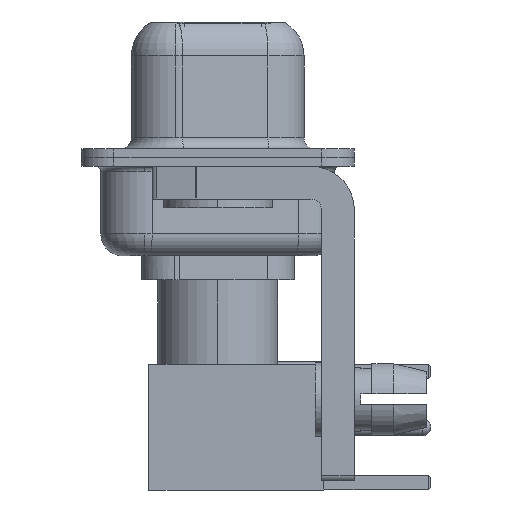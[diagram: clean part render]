
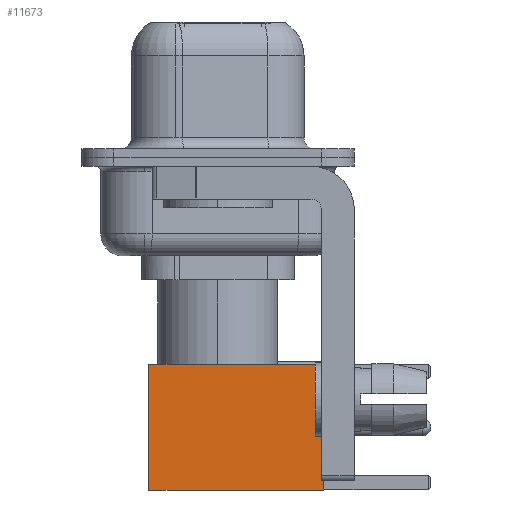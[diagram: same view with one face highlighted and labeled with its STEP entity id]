
A CAD part, left-side view. The second image highlights one B-rep face of the part: STEP entity #11673.
In plain terms, the highlighted face is planar.
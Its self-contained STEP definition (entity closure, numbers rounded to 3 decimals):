
#949 = EDGE_CURVE ( 'NONE', #5847, #16238, #15309, .T. ) ;
#1483 = VERTEX_POINT ( 'NONE', #9457 ) ;
#2577 = CARTESIAN_POINT ( 'NONE',  ( 2.875, 2.875, 0. ) ) ;
#3178 = AXIS2_PLACEMENT_3D ( 'NONE', #21093, #12056, #19308 ) ;
#4596 = EDGE_CURVE ( 'NONE', #1483, #5847, #5017, .T. ) ;
#5017 = LINE ( 'NONE', #12324, #17441 ) ;
#5847 = VERTEX_POINT ( 'NONE', #8816 ) ;
#6822 = ORIENTED_EDGE ( 'NONE', *, *, #949, .F. ) ;
#7757 = LINE ( 'NONE', #15028, #9255 ) ;
#8816 = CARTESIAN_POINT ( 'NONE',  ( -2.875, 2.875, 8. ) ) ;
#9255 = VECTOR ( 'NONE', #9787, 1000. ) ;
#9457 = CARTESIAN_POINT ( 'NONE',  ( 2.875, 2.875, 8. ) ) ;
#9787 = DIRECTION ( 'NONE',  ( -1., 0., 0. ) ) ;
#10222 = EDGE_CURVE ( 'NONE', #1483, #11924, #11119, .T. ) ;
#10502 = EDGE_CURVE ( 'NONE', #11924, #16238, #7757, .T. ) ;
#11119 = LINE ( 'NONE', #18610, #15742 ) ;
#11673 = ADVANCED_FACE ( 'NONE', ( #21337 ), #23130, .T. ) ;
#11924 = VERTEX_POINT ( 'NONE', #2577 ) ;
#12056 = DIRECTION ( 'NONE',  ( 0., 1., 0. ) ) ;
#12324 = CARTESIAN_POINT ( 'NONE',  ( 0., 2.875, 8. ) ) ;
#13597 = ORIENTED_EDGE ( 'NONE', *, *, #10502, .T. ) ;
#14187 = CARTESIAN_POINT ( 'NONE',  ( -2.875, 2.875, 0. ) ) ;
#15028 = CARTESIAN_POINT ( 'NONE',  ( 0., 2.875, 0. ) ) ;
#15309 = LINE ( 'NONE', #16983, #20272 ) ;
#15742 = VECTOR ( 'NONE', #16346, 1000. ) ;
#15828 = EDGE_LOOP ( 'NONE', ( #17314, #13597, #6822, #17850 ) ) ;
#16238 = VERTEX_POINT ( 'NONE', #14187 ) ;
#16346 = DIRECTION ( 'NONE',  ( 0., 0., -1. ) ) ;
#16983 = CARTESIAN_POINT ( 'NONE',  ( -2.875, 2.875, 0. ) ) ;
#17314 = ORIENTED_EDGE ( 'NONE', *, *, #10222, .T. ) ;
#17441 = VECTOR ( 'NONE', #19584, 1000. ) ;
#17850 = ORIENTED_EDGE ( 'NONE', *, *, #4596, .F. ) ;
#18610 = CARTESIAN_POINT ( 'NONE',  ( 2.875, 2.875, 0. ) ) ;
#18770 = DIRECTION ( 'NONE',  ( 0., 0., -1. ) ) ;
#19308 = DIRECTION ( 'NONE',  ( 0., 0., 1. ) ) ;
#19584 = DIRECTION ( 'NONE',  ( -1., 0., 0. ) ) ;
#20272 = VECTOR ( 'NONE', #18770, 1000. ) ;
#21093 = CARTESIAN_POINT ( 'NONE',  ( 2.875, 2.875, 0. ) ) ;
#21337 = FACE_OUTER_BOUND ( 'NONE', #15828, .T. ) ;
#23130 = PLANE ( 'NONE',  #3178 ) ;
